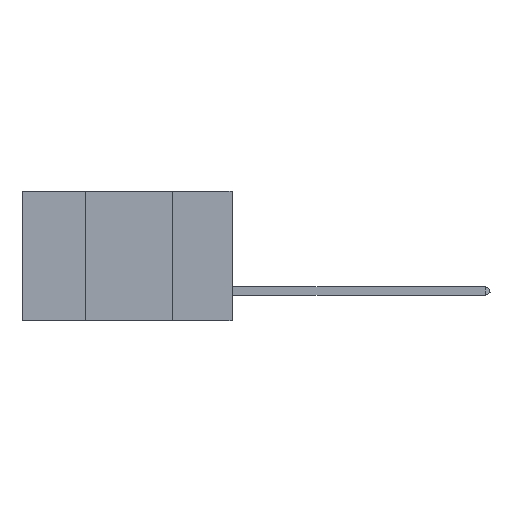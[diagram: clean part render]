
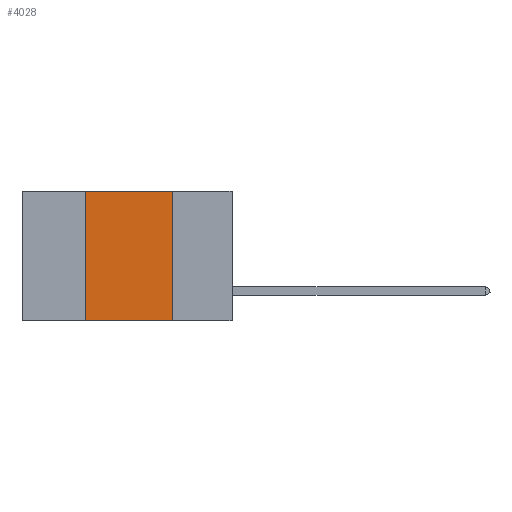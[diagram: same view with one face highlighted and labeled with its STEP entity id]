
A CAD part, left-side view. The second image highlights one B-rep face of the part: STEP entity #4028.
In plain terms, the highlighted planar face has unit normal (-1, 0, 0).
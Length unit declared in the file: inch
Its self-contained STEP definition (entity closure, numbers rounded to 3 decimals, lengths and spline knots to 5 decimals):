
#343 = VECTOR ( 'NONE', #4241, 39.37008 ) ;
#4028 = ADVANCED_FACE ( 'NONE', ( #8667 ), #47998, .F. ) ;
#4241 = DIRECTION ( 'NONE',  ( 0., 0., -1. ) ) ;
#6267 = ORIENTED_EDGE ( 'NONE', *, *, #12008, .F. ) ;
#7197 = CARTESIAN_POINT ( 'NONE',  ( 0., 0.6, -0.37 ) ) ;
#7743 = EDGE_CURVE ( 'NONE', #13451, #36938, #40093, .T. ) ;
#8667 = FACE_OUTER_BOUND ( 'NONE', #20140, .T. ) ;
#9449 = VECTOR ( 'NONE', #36689, 39.37008 ) ;
#9896 = CARTESIAN_POINT ( 'NONE',  ( 0., 0.17, -0.37 ) ) ;
#10966 = CARTESIAN_POINT ( 'NONE',  ( 0., 0.42, -0.37 ) ) ;
#12008 = EDGE_CURVE ( 'NONE', #46487, #13451, #14578, .T. ) ;
#13451 = VERTEX_POINT ( 'NONE', #41515 ) ;
#14578 = LINE ( 'NONE', #42826, #46791 ) ;
#20140 = EDGE_LOOP ( 'NONE', ( #35801, #26702, #6267, #44551 ) ) ;
#22244 = DIRECTION ( 'NONE',  ( 1., 0., 0. ) ) ;
#22605 = CARTESIAN_POINT ( 'NONE',  ( 0., 0.17, 0. ) ) ;
#26616 = DIRECTION ( 'NONE',  ( 0., -1., 0. ) ) ;
#26702 = ORIENTED_EDGE ( 'NONE', *, *, #7743, .F. ) ;
#27449 = VERTEX_POINT ( 'NONE', #9896 ) ;
#29920 = DIRECTION ( 'NONE',  ( 0., 0., -1. ) ) ;
#30062 = CARTESIAN_POINT ( 'NONE',  ( 0., 0.6, 0. ) ) ;
#30927 = DIRECTION ( 'NONE',  ( 0., 0., 1. ) ) ;
#32174 = EDGE_CURVE ( 'NONE', #46487, #27449, #48115, .T. ) ;
#33554 = AXIS2_PLACEMENT_3D ( 'NONE', #37152, #22244, #29920 ) ;
#35801 = ORIENTED_EDGE ( 'NONE', *, *, #40277, .F. ) ;
#36689 = DIRECTION ( 'NONE',  ( 0., -1., 0. ) ) ;
#36938 = VERTEX_POINT ( 'NONE', #22605 ) ;
#37152 = CARTESIAN_POINT ( 'NONE',  ( 0., 0.6, 0. ) ) ;
#40093 = LINE ( 'NONE', #30062, #40648 ) ;
#40277 = EDGE_CURVE ( 'NONE', #36938, #27449, #43109, .T. ) ;
#40648 = VECTOR ( 'NONE', #26616, 39.37008 ) ;
#41515 = CARTESIAN_POINT ( 'NONE',  ( 0., 0.42, 0. ) ) ;
#42826 = CARTESIAN_POINT ( 'NONE',  ( 0., 0.42, 0. ) ) ;
#43109 = LINE ( 'NONE', #45180, #343 ) ;
#44551 = ORIENTED_EDGE ( 'NONE', *, *, #32174, .T. ) ;
#45180 = CARTESIAN_POINT ( 'NONE',  ( 0., 0.17, 0. ) ) ;
#46487 = VERTEX_POINT ( 'NONE', #10966 ) ;
#46791 = VECTOR ( 'NONE', #30927, 39.37008 ) ;
#47998 = PLANE ( 'NONE',  #33554 ) ;
#48115 = LINE ( 'NONE', #7197, #9449 ) ;
